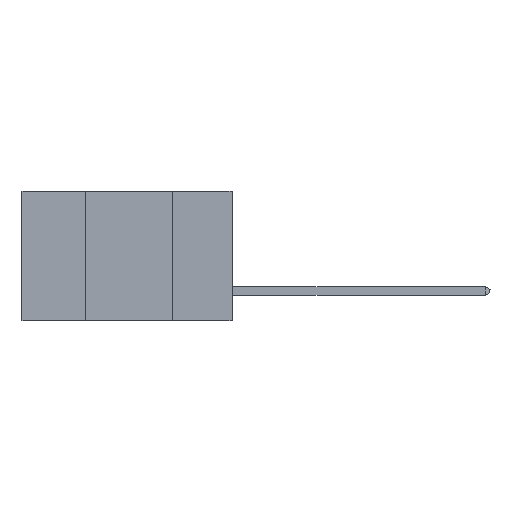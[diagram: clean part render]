
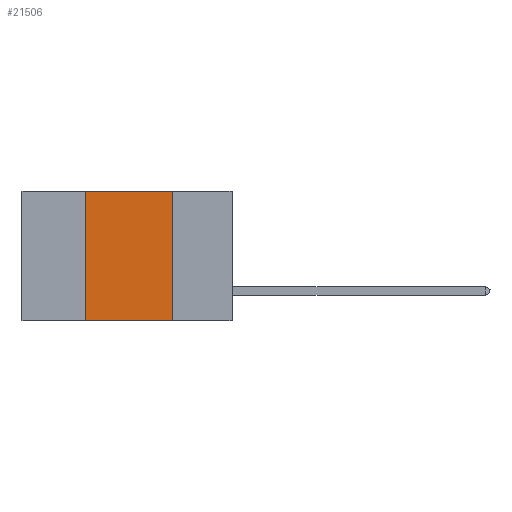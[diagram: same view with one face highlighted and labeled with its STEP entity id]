
A CAD part, left-side view. The second image highlights one B-rep face of the part: STEP entity #21506.
In plain terms, the highlighted planar face has unit normal (-1, 0, 0).
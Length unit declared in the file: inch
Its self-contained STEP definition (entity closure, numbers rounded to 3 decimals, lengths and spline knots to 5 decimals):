
#616 = VERTEX_POINT ( 'NONE', #6317 ) ;
#823 = ORIENTED_EDGE ( 'NONE', *, *, #37009, .F. ) ;
#2879 = DIRECTION ( 'NONE',  ( 0., -1., 0. ) ) ;
#2930 = VECTOR ( 'NONE', #2879, 39.37008 ) ;
#3900 = CARTESIAN_POINT ( 'NONE',  ( 0., 0.17, -0.37 ) ) ;
#5126 = ORIENTED_EDGE ( 'NONE', *, *, #10442, .T. ) ;
#5577 = CARTESIAN_POINT ( 'NONE',  ( 0., 0.6, -0.37 ) ) ;
#5837 = DIRECTION ( 'NONE',  ( 0., 0., -1. ) ) ;
#6317 = CARTESIAN_POINT ( 'NONE',  ( 0., 0.17, 0. ) ) ;
#8403 = DIRECTION ( 'NONE',  ( 0., 0., 1. ) ) ;
#9412 = VECTOR ( 'NONE', #8403, 39.37008 ) ;
#9448 = VERTEX_POINT ( 'NONE', #38062 ) ;
#10442 = EDGE_CURVE ( 'NONE', #33126, #30986, #30364, .T. ) ;
#17648 = LINE ( 'NONE', #29833, #9412 ) ;
#20585 = LINE ( 'NONE', #29160, #33951 ) ;
#21208 = ORIENTED_EDGE ( 'NONE', *, *, #28412, .F. ) ;
#21506 = ADVANCED_FACE ( 'NONE', ( #37327 ), #29469, .F. ) ;
#24454 = DIRECTION ( 'NONE',  ( 0., -1., 0. ) ) ;
#25042 = LINE ( 'NONE', #36600, #37949 ) ;
#25555 = AXIS2_PLACEMENT_3D ( 'NONE', #28739, #39147, #5837 ) ;
#28412 = EDGE_CURVE ( 'NONE', #33126, #9448, #17648, .T. ) ;
#28739 = CARTESIAN_POINT ( 'NONE',  ( 0., 0.6, 0. ) ) ;
#29160 = CARTESIAN_POINT ( 'NONE',  ( 0., 0.17, 0. ) ) ;
#29469 = PLANE ( 'NONE',  #25555 ) ;
#29707 = CARTESIAN_POINT ( 'NONE',  ( 0., 0.42, -0.37 ) ) ;
#29833 = CARTESIAN_POINT ( 'NONE',  ( 0., 0.42, 0. ) ) ;
#30364 = LINE ( 'NONE', #5577, #2930 ) ;
#30986 = VERTEX_POINT ( 'NONE', #3900 ) ;
#31785 = EDGE_LOOP ( 'NONE', ( #36469, #823, #21208, #5126 ) ) ;
#32996 = DIRECTION ( 'NONE',  ( 0., 0., -1. ) ) ;
#33126 = VERTEX_POINT ( 'NONE', #29707 ) ;
#33951 = VECTOR ( 'NONE', #32996, 39.37008 ) ;
#36469 = ORIENTED_EDGE ( 'NONE', *, *, #38594, .F. ) ;
#36600 = CARTESIAN_POINT ( 'NONE',  ( 0., 0.6, 0. ) ) ;
#37009 = EDGE_CURVE ( 'NONE', #9448, #616, #25042, .T. ) ;
#37327 = FACE_OUTER_BOUND ( 'NONE', #31785, .T. ) ;
#37949 = VECTOR ( 'NONE', #24454, 39.37008 ) ;
#38062 = CARTESIAN_POINT ( 'NONE',  ( 0., 0.42, 0. ) ) ;
#38594 = EDGE_CURVE ( 'NONE', #616, #30986, #20585, .T. ) ;
#39147 = DIRECTION ( 'NONE',  ( 1., 0., 0. ) ) ;
